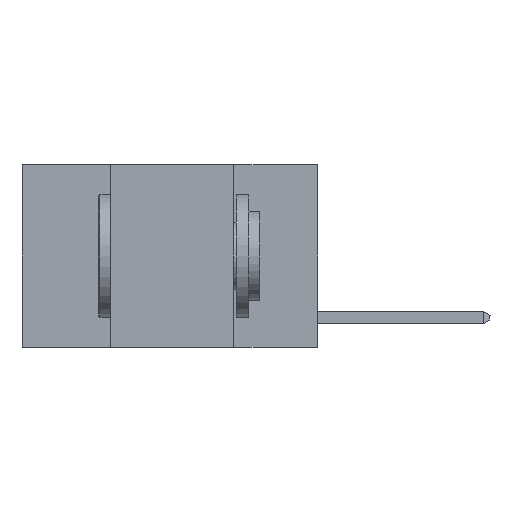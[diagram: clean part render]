
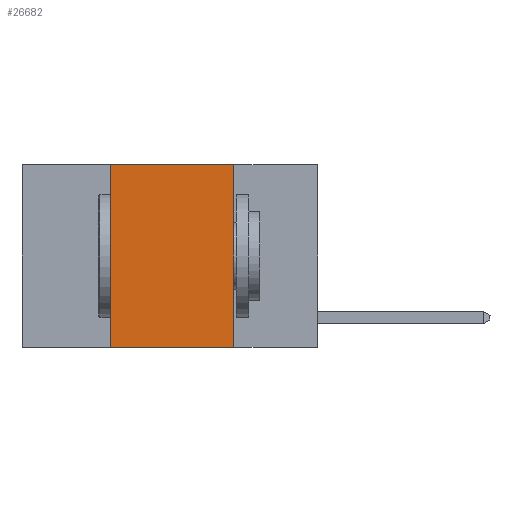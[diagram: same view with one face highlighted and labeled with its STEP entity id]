
A CAD part, left-side view. The second image highlights one B-rep face of the part: STEP entity #26682.
In plain terms, the highlighted planar face has unit normal (-1, 0, 0).
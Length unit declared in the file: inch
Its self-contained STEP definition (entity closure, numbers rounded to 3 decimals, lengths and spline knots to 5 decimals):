
#227 = DIRECTION ( 'NONE',  ( 0., -1., 0. ) ) ;
#479 = EDGE_CURVE ( 'NONE', #20597, #2543, #19146, .T. ) ;
#957 = VERTEX_POINT ( 'NONE', #25698 ) ;
#1891 = EDGE_CURVE ( 'NONE', #20597, #957, #12022, .T. ) ;
#2543 = VERTEX_POINT ( 'NONE', #17357 ) ;
#2681 = CARTESIAN_POINT ( 'NONE',  ( 0., 0.42, -0.37 ) ) ;
#3396 = CARTESIAN_POINT ( 'NONE',  ( 0., 0.17, 0. ) ) ;
#3750 = VECTOR ( 'NONE', #17683, 39.37008 ) ;
#4867 = AXIS2_PLACEMENT_3D ( 'NONE', #12671, #15030, #21105 ) ;
#8816 = ORIENTED_EDGE ( 'NONE', *, *, #19790, .F. ) ;
#9052 = EDGE_CURVE ( 'NONE', #11992, #2543, #10072, .T. ) ;
#9537 = DIRECTION ( 'NONE',  ( 0., 0., 1. ) ) ;
#9791 = CARTESIAN_POINT ( 'NONE',  ( 0., 0.6, 0. ) ) ;
#10072 = LINE ( 'NONE', #18521, #26384 ) ;
#11992 = VERTEX_POINT ( 'NONE', #3396 ) ;
#12022 = LINE ( 'NONE', #26547, #17175 ) ;
#12671 = CARTESIAN_POINT ( 'NONE',  ( 0., 0.6, 0. ) ) ;
#13457 = EDGE_LOOP ( 'NONE', ( #17233, #8816, #27301, #26218 ) ) ;
#15030 = DIRECTION ( 'NONE',  ( 1., 0., 0. ) ) ;
#16013 = LINE ( 'NONE', #9791, #3750 ) ;
#16443 = FACE_OUTER_BOUND ( 'NONE', #13457, .T. ) ;
#16642 = CARTESIAN_POINT ( 'NONE',  ( 0., 0.6, -0.37 ) ) ;
#17175 = VECTOR ( 'NONE', #9537, 39.37008 ) ;
#17233 = ORIENTED_EDGE ( 'NONE', *, *, #9052, .F. ) ;
#17357 = CARTESIAN_POINT ( 'NONE',  ( 0., 0.17, -0.37 ) ) ;
#17683 = DIRECTION ( 'NONE',  ( 0., -1., 0. ) ) ;
#18521 = CARTESIAN_POINT ( 'NONE',  ( 0., 0.17, 0. ) ) ;
#19146 = LINE ( 'NONE', #16642, #25031 ) ;
#19790 = EDGE_CURVE ( 'NONE', #957, #11992, #16013, .T. ) ;
#20597 = VERTEX_POINT ( 'NONE', #2681 ) ;
#21105 = DIRECTION ( 'NONE',  ( 0., 0., -1. ) ) ;
#21245 = PLANE ( 'NONE',  #4867 ) ;
#25031 = VECTOR ( 'NONE', #227, 39.37008 ) ;
#25698 = CARTESIAN_POINT ( 'NONE',  ( 0., 0.42, 0. ) ) ;
#26218 = ORIENTED_EDGE ( 'NONE', *, *, #479, .T. ) ;
#26384 = VECTOR ( 'NONE', #27223, 39.37008 ) ;
#26547 = CARTESIAN_POINT ( 'NONE',  ( 0., 0.42, 0. ) ) ;
#26682 = ADVANCED_FACE ( 'NONE', ( #16443 ), #21245, .F. ) ;
#27223 = DIRECTION ( 'NONE',  ( 0., 0., -1. ) ) ;
#27301 = ORIENTED_EDGE ( 'NONE', *, *, #1891, .F. ) ;
